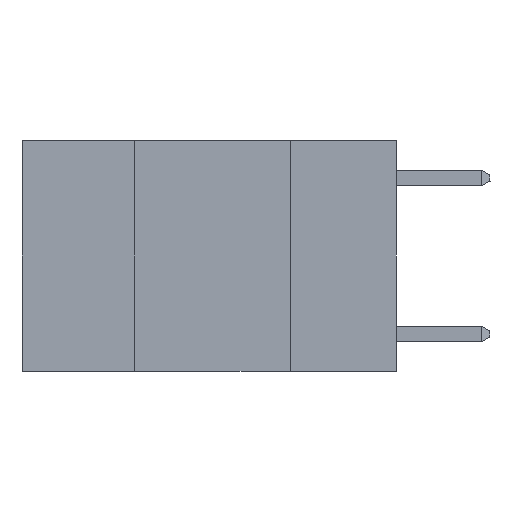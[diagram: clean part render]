
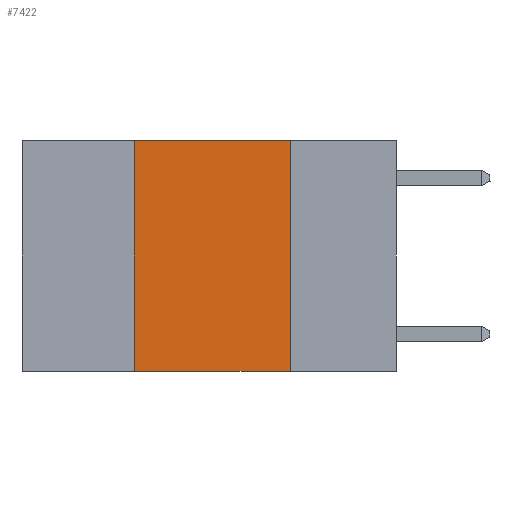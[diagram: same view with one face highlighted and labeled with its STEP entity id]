
A CAD part, left-side view. The second image highlights one B-rep face of the part: STEP entity #7422.
In plain terms, the highlighted planar face has unit normal (-1, 0, 0).
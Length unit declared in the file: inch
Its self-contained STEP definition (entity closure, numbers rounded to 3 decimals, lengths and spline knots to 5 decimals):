
#439 = LINE ( 'NONE', #1568, #6580 ) ;
#1568 = CARTESIAN_POINT ( 'NONE',  ( 0., 0.6, 0. ) ) ;
#1805 = DIRECTION ( 'NONE',  ( 0., -1., 0. ) ) ;
#2621 = EDGE_CURVE ( 'NONE', #12314, #12165, #2872, .T. ) ;
#2872 = LINE ( 'NONE', #7599, #4993 ) ;
#2913 = VECTOR ( 'NONE', #4192, 39.37008 ) ;
#3019 = DIRECTION ( 'NONE',  ( 0., 0., 1. ) ) ;
#3472 = EDGE_CURVE ( 'NONE', #6664, #12314, #439, .T. ) ;
#3486 = CARTESIAN_POINT ( 'NONE',  ( 0., 0.42, 0. ) ) ;
#4063 = CARTESIAN_POINT ( 'NONE',  ( 0., 0.42, 0. ) ) ;
#4116 = EDGE_CURVE ( 'NONE', #7354, #6664, #9355, .T. ) ;
#4192 = DIRECTION ( 'NONE',  ( 0., -1., 0. ) ) ;
#4993 = VECTOR ( 'NONE', #7542, 39.37008 ) ;
#5221 = DIRECTION ( 'NONE',  ( 0., 0., -1. ) ) ;
#5233 = DIRECTION ( 'NONE',  ( 1., 0., 0. ) ) ;
#5279 = PLANE ( 'NONE',  #6897 ) ;
#5331 = CARTESIAN_POINT ( 'NONE',  ( 0., 0.6, 0. ) ) ;
#6000 = CARTESIAN_POINT ( 'NONE',  ( 0., 0.42, -0.37 ) ) ;
#6580 = VECTOR ( 'NONE', #1805, 39.37008 ) ;
#6584 = VECTOR ( 'NONE', #3019, 39.37008 ) ;
#6664 = VERTEX_POINT ( 'NONE', #4063 ) ;
#6665 = FACE_OUTER_BOUND ( 'NONE', #10226, .T. ) ;
#6683 = ORIENTED_EDGE ( 'NONE', *, *, #2621, .F. ) ;
#6897 = AXIS2_PLACEMENT_3D ( 'NONE', #5331, #5233, #5221 ) ;
#7278 = CARTESIAN_POINT ( 'NONE',  ( 0., 0.6, -0.37 ) ) ;
#7354 = VERTEX_POINT ( 'NONE', #6000 ) ;
#7422 = ADVANCED_FACE ( 'NONE', ( #6665 ), #5279, .F. ) ;
#7542 = DIRECTION ( 'NONE',  ( 0., 0., -1. ) ) ;
#7599 = CARTESIAN_POINT ( 'NONE',  ( 0., 0.17, 0. ) ) ;
#7998 = EDGE_CURVE ( 'NONE', #7354, #12165, #8457, .T. ) ;
#8457 = LINE ( 'NONE', #7278, #2913 ) ;
#9292 = ORIENTED_EDGE ( 'NONE', *, *, #7998, .T. ) ;
#9355 = LINE ( 'NONE', #3486, #6584 ) ;
#10142 = CARTESIAN_POINT ( 'NONE',  ( 0., 0.17, 0. ) ) ;
#10226 = EDGE_LOOP ( 'NONE', ( #6683, #11833, #13207, #9292 ) ) ;
#10948 = CARTESIAN_POINT ( 'NONE',  ( 0., 0.17, -0.37 ) ) ;
#11833 = ORIENTED_EDGE ( 'NONE', *, *, #3472, .F. ) ;
#12165 = VERTEX_POINT ( 'NONE', #10948 ) ;
#12314 = VERTEX_POINT ( 'NONE', #10142 ) ;
#13207 = ORIENTED_EDGE ( 'NONE', *, *, #4116, .F. ) ;
